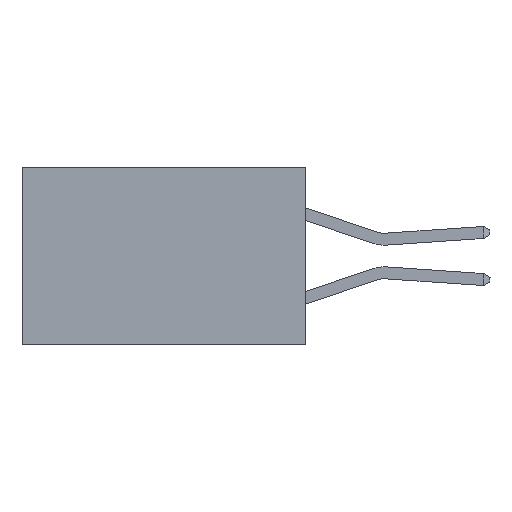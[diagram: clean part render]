
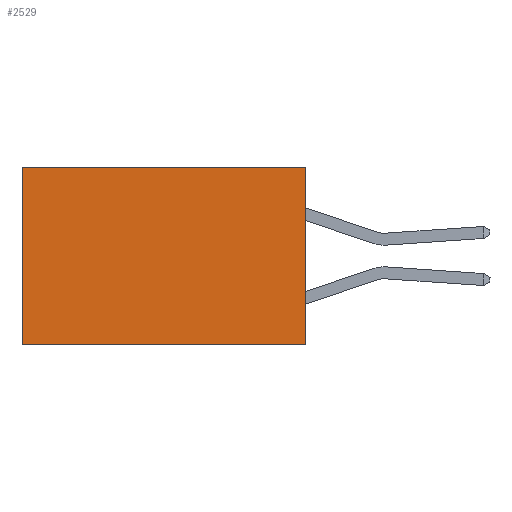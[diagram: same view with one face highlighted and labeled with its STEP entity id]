
A CAD part, left-side view. The second image highlights one B-rep face of the part: STEP entity #2529.
In plain terms, the highlighted planar face has unit normal (-1, 0, 0).
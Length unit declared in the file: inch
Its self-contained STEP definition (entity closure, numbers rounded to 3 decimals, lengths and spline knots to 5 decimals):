
#121 = VECTOR ( 'NONE', #3872, 39.37008 ) ;
#186 = CARTESIAN_POINT ( 'NONE',  ( 0.277, 0., -0.37 ) ) ;
#205 = VECTOR ( 'NONE', #6503, 39.37008 ) ;
#254 = CARTESIAN_POINT ( 'NONE',  ( 0.277, 0., 0. ) ) ;
#278 = VERTEX_POINT ( 'NONE', #254 ) ;
#339 = LINE ( 'NONE', #186, #121 ) ;
#746 = VECTOR ( 'NONE', #5079, 39.37008 ) ;
#1720 = EDGE_CURVE ( 'NONE', #278, #6894, #4698, .T. ) ;
#2137 = CARTESIAN_POINT ( 'NONE',  ( 0.277, 0.59, -0.37 ) ) ;
#2425 = CARTESIAN_POINT ( 'NONE',  ( 0.277, 0.59, -0.37 ) ) ;
#2529 = ADVANCED_FACE ( 'NONE', ( #3418 ), #5897, .F. ) ;
#2874 = LINE ( 'NONE', #2137, #205 ) ;
#3418 = FACE_OUTER_BOUND ( 'NONE', #7674, .T. ) ;
#3515 = ORIENTED_EDGE ( 'NONE', *, *, #4616, .T. ) ;
#3774 = VERTEX_POINT ( 'NONE', #2425 ) ;
#3872 = DIRECTION ( 'NONE',  ( 0., 1., 0. ) ) ;
#4187 = VERTEX_POINT ( 'NONE', #4470 ) ;
#4190 = LINE ( 'NONE', #5810, #4428 ) ;
#4428 = VECTOR ( 'NONE', #5864, 39.37008 ) ;
#4470 = CARTESIAN_POINT ( 'NONE',  ( 0.277, 0.59, 0. ) ) ;
#4616 = EDGE_CURVE ( 'NONE', #278, #4187, #4190, .T. ) ;
#4698 = LINE ( 'NONE', #7245, #746 ) ;
#5079 = DIRECTION ( 'NONE',  ( 0., 0., -1. ) ) ;
#5810 = CARTESIAN_POINT ( 'NONE',  ( 0.277, 0., 0. ) ) ;
#5864 = DIRECTION ( 'NONE',  ( 0., 1., 0. ) ) ;
#5897 = PLANE ( 'NONE',  #9226 ) ;
#5940 = DIRECTION ( 'NONE',  ( 1., 0., 0. ) ) ;
#6047 = ORIENTED_EDGE ( 'NONE', *, *, #1720, .F. ) ;
#6293 = ORIENTED_EDGE ( 'NONE', *, *, #7870, .F. ) ;
#6503 = DIRECTION ( 'NONE',  ( 0., 0., -1. ) ) ;
#6618 = ORIENTED_EDGE ( 'NONE', *, *, #8906, .T. ) ;
#6894 = VERTEX_POINT ( 'NONE', #7638 ) ;
#7245 = CARTESIAN_POINT ( 'NONE',  ( 0.277, 0., -0.37 ) ) ;
#7638 = CARTESIAN_POINT ( 'NONE',  ( 0.277, 0., -0.37 ) ) ;
#7674 = EDGE_LOOP ( 'NONE', ( #6618, #6293, #6047, #3515 ) ) ;
#7870 = EDGE_CURVE ( 'NONE', #6894, #3774, #339, .T. ) ;
#7946 = CARTESIAN_POINT ( 'NONE',  ( 0.277, 0., -0.37 ) ) ;
#8595 = DIRECTION ( 'NONE',  ( 0., 0., -1. ) ) ;
#8906 = EDGE_CURVE ( 'NONE', #4187, #3774, #2874, .T. ) ;
#9226 = AXIS2_PLACEMENT_3D ( 'NONE', #7946, #5940, #8595 ) ;
